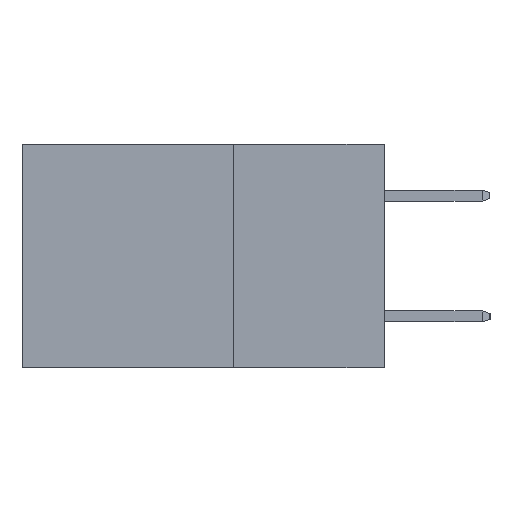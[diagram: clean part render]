
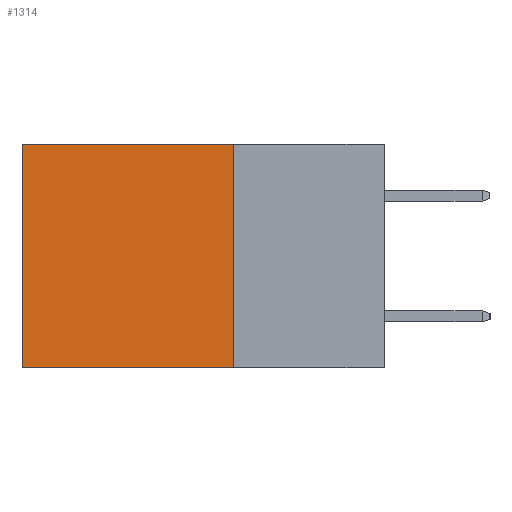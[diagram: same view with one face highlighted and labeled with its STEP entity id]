
A CAD part, left-side view. The second image highlights one B-rep face of the part: STEP entity #1314.
In plain terms, the highlighted planar face has unit normal (-1, 0, 0).
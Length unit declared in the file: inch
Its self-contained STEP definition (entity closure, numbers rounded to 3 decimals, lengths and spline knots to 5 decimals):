
#15 = VECTOR ( 'NONE', #10405, 39.37008 ) ;
#248 = VERTEX_POINT ( 'NONE', #4786 ) ;
#275 = CARTESIAN_POINT ( 'NONE',  ( 0.2615, 0.25, -0.37 ) ) ;
#342 = LINE ( 'NONE', #275, #15 ) ;
#430 = DIRECTION ( 'NONE',  ( 0., 1., 0. ) ) ;
#1163 = VECTOR ( 'NONE', #2011, 39.37008 ) ;
#1314 = ADVANCED_FACE ( 'NONE', ( #9828 ), #5295, .F. ) ;
#1737 = EDGE_LOOP ( 'NONE', ( #2575, #9668, #9638, #9883 ) ) ;
#2011 = DIRECTION ( 'NONE',  ( 0., 0., -1. ) ) ;
#2090 = CARTESIAN_POINT ( 'NONE',  ( 0.2615, 0.25, -0.37 ) ) ;
#2477 = EDGE_CURVE ( 'NONE', #5646, #5659, #342, .T. ) ;
#2575 = ORIENTED_EDGE ( 'NONE', *, *, #10139, .T. ) ;
#2802 = EDGE_CURVE ( 'NONE', #5659, #248, #6667, .T. ) ;
#4777 = CARTESIAN_POINT ( 'NONE',  ( 0.2615, 0.6, 0. ) ) ;
#4786 = CARTESIAN_POINT ( 'NONE',  ( 0.2615, 0.6, -0.37 ) ) ;
#5105 = DIRECTION ( 'NONE',  ( 0., 0., -1. ) ) ;
#5136 = DIRECTION ( 'NONE',  ( 1., 0., 0. ) ) ;
#5295 = PLANE ( 'NONE',  #8383 ) ;
#5646 = VERTEX_POINT ( 'NONE', #6716 ) ;
#5659 = VERTEX_POINT ( 'NONE', #2090 ) ;
#6129 = LINE ( 'NONE', #11224, #10593 ) ;
#6232 = LINE ( 'NONE', #11629, #1163 ) ;
#6416 = CARTESIAN_POINT ( 'NONE',  ( 0.2615, 0.25, -0.37 ) ) ;
#6667 = LINE ( 'NONE', #6680, #10850 ) ;
#6680 = CARTESIAN_POINT ( 'NONE',  ( 0.2615, 0.25, -0.37 ) ) ;
#6716 = CARTESIAN_POINT ( 'NONE',  ( 0.2615, 0.25, 0. ) ) ;
#8205 = EDGE_CURVE ( 'NONE', #5646, #10032, #6129, .T. ) ;
#8383 = AXIS2_PLACEMENT_3D ( 'NONE', #6416, #5136, #5105 ) ;
#8409 = DIRECTION ( 'NONE',  ( 0., 1., 0. ) ) ;
#9638 = ORIENTED_EDGE ( 'NONE', *, *, #2477, .F. ) ;
#9668 = ORIENTED_EDGE ( 'NONE', *, *, #2802, .F. ) ;
#9828 = FACE_OUTER_BOUND ( 'NONE', #1737, .T. ) ;
#9883 = ORIENTED_EDGE ( 'NONE', *, *, #8205, .T. ) ;
#10032 = VERTEX_POINT ( 'NONE', #4777 ) ;
#10139 = EDGE_CURVE ( 'NONE', #10032, #248, #6232, .T. ) ;
#10405 = DIRECTION ( 'NONE',  ( 0., 0., -1. ) ) ;
#10593 = VECTOR ( 'NONE', #430, 39.37008 ) ;
#10850 = VECTOR ( 'NONE', #8409, 39.37008 ) ;
#11224 = CARTESIAN_POINT ( 'NONE',  ( 0.2615, 0.25, 0. ) ) ;
#11629 = CARTESIAN_POINT ( 'NONE',  ( 0.2615, 0.6, -0.37 ) ) ;
